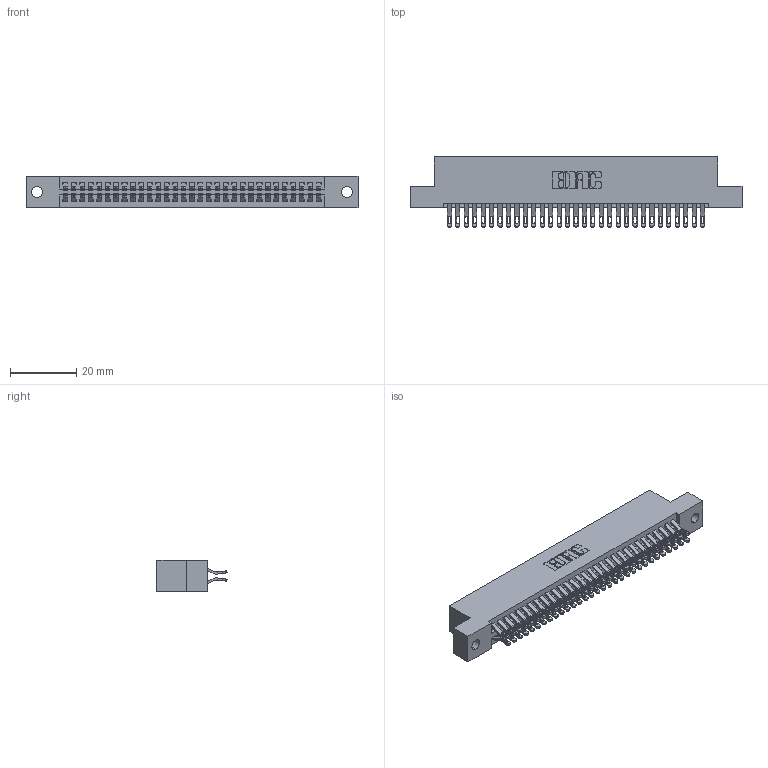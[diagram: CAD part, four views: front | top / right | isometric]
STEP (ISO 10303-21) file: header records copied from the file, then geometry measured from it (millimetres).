
FILE_DESCRIPTION (( 'STEP AP203' ), '1' );
FILE_NAME ('345-062-555-202.STEP', '2018-09-27T16:21:29', ( '' ), ( '' ), 'SwSTEP 2.0', 'SolidWorks 2016', '' );
FILE_SCHEMA (( 'CONFIG_CONTROL_DESIGN' ));
Length unit declared in the file: inch
Products named in the file (3): 345 Part_Flush Mounting Lugs - 0.128 Dia; 345-062-555-202; 345-292-001_555 Tail
Assembly tree (63 placements, depth 2):
  345-062-555-202
    345 Part_Flush Mounting Lugs - 0.128 Dia
    345-292-001_555 Tail  x62
Bounding box: 99.95 x 21.13 x 9.4 mm (x, y, z)
Volume: 9750.2 mm3; surface area: 14552.1 mm2
Topology: 63 solids, 63 shells, 3598 faces, 11315 edges, 7542 vertices
Faces by surface type: plane 2002, cylinder 1596
Entity records: 26133 total; most frequent: CARTESIAN_POINT 4426, ORIENTED_EDGE 4330, DIRECTION 3885, EDGE_CURVE 2165, VECTOR 1889, LINE 1889, VERTEX_POINT 1442, AXIS2_PLACEMENT_3D 998
